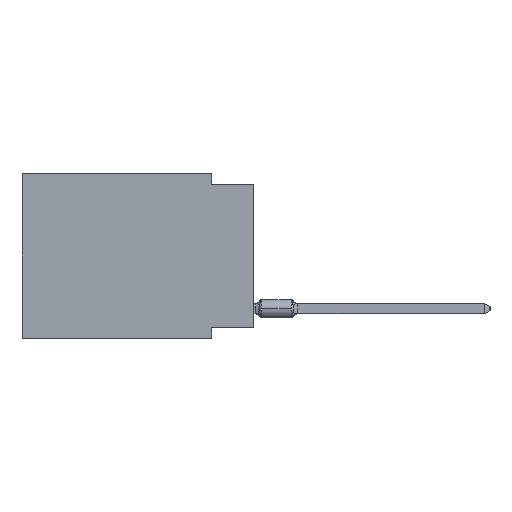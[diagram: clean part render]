
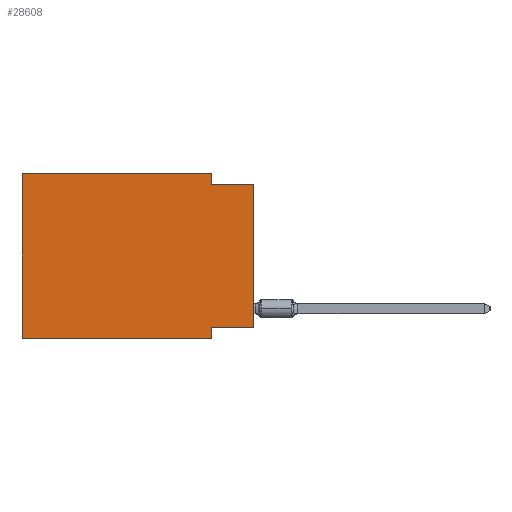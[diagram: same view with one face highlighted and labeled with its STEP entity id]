
A CAD part, left-side view. The second image highlights one B-rep face of the part: STEP entity #28608.
In plain terms, the highlighted planar face has unit normal (-1, 0, 0).
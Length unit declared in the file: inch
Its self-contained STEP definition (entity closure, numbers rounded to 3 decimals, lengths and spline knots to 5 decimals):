
#1460 = ORIENTED_EDGE ( 'NONE', *, *, #8875, .F. ) ;
#2467 = CARTESIAN_POINT ( 'NONE',  ( 0., 0.1, 0. ) ) ;
#2951 = VECTOR ( 'NONE', #33342, 39.37008 ) ;
#3964 = ORIENTED_EDGE ( 'NONE', *, *, #6357, .T. ) ;
#4202 = DIRECTION ( 'NONE',  ( 0., -1., 0. ) ) ;
#4640 = VECTOR ( 'NONE', #26153, 39.37008 ) ;
#4978 = VERTEX_POINT ( 'NONE', #22599 ) ;
#5071 = CARTESIAN_POINT ( 'NONE',  ( 0., 0.1, -0.39 ) ) ;
#5503 = LINE ( 'NONE', #30971, #20726 ) ;
#5688 = VECTOR ( 'NONE', #14243, 39.37008 ) ;
#6357 = EDGE_CURVE ( 'NONE', #12077, #12514, #19902, .T. ) ;
#6684 = CARTESIAN_POINT ( 'NONE',  ( 0., 0.55, 0. ) ) ;
#7269 = LINE ( 'NONE', #5071, #28558 ) ;
#7432 = PLANE ( 'NONE',  #23511 ) ;
#7542 = CARTESIAN_POINT ( 'NONE',  ( 0., 0.1, -0.39 ) ) ;
#7675 = ORIENTED_EDGE ( 'NONE', *, *, #27380, .F. ) ;
#8429 = CARTESIAN_POINT ( 'NONE',  ( 0., 0., -0.365 ) ) ;
#8778 = LINE ( 'NONE', #22241, #9567 ) ;
#8875 = EDGE_CURVE ( 'NONE', #13925, #28356, #27230, .T. ) ;
#9567 = VECTOR ( 'NONE', #32204, 39.37008 ) ;
#9795 = CARTESIAN_POINT ( 'NONE',  ( 0., 0.55, 0. ) ) ;
#10225 = ORIENTED_EDGE ( 'NONE', *, *, #12659, .T. ) ;
#10295 = DIRECTION ( 'NONE',  ( 0., 0., -1. ) ) ;
#10405 = ORIENTED_EDGE ( 'NONE', *, *, #28668, .F. ) ;
#10538 = CARTESIAN_POINT ( 'NONE',  ( 0., 0., -0.025 ) ) ;
#10794 = EDGE_CURVE ( 'NONE', #19564, #29018, #8778, .T. ) ;
#11011 = CARTESIAN_POINT ( 'NONE',  ( 0., 0.55, -0.39 ) ) ;
#12077 = VERTEX_POINT ( 'NONE', #11011 ) ;
#12514 = VERTEX_POINT ( 'NONE', #7542 ) ;
#12576 = VECTOR ( 'NONE', #4202, 39.37008 ) ;
#12659 = EDGE_CURVE ( 'NONE', #4978, #28356, #5503, .T. ) ;
#13331 = LINE ( 'NONE', #8429, #4640 ) ;
#13606 = CARTESIAN_POINT ( 'NONE',  ( 0., 0.55, 0. ) ) ;
#13925 = VERTEX_POINT ( 'NONE', #26215 ) ;
#13953 = LINE ( 'NONE', #13606, #26763 ) ;
#14243 = DIRECTION ( 'NONE',  ( 0., -1., 0. ) ) ;
#14896 = VERTEX_POINT ( 'NONE', #31505 ) ;
#15834 = ORIENTED_EDGE ( 'NONE', *, *, #10794, .F. ) ;
#15968 = DIRECTION ( 'NONE',  ( 0., 0., 1. ) ) ;
#16368 = EDGE_CURVE ( 'NONE', #12077, #19564, #13953, .T. ) ;
#17104 = CARTESIAN_POINT ( 'NONE',  ( 0., 0., -0.025 ) ) ;
#17888 = FACE_OUTER_BOUND ( 'NONE', #33219, .T. ) ;
#19564 = VERTEX_POINT ( 'NONE', #6684 ) ;
#19902 = LINE ( 'NONE', #27339, #12576 ) ;
#20713 = LINE ( 'NONE', #33001, #2951 ) ;
#20726 = VECTOR ( 'NONE', #31316, 39.37008 ) ;
#22241 = CARTESIAN_POINT ( 'NONE',  ( 0., 0.55, 0. ) ) ;
#22428 = DIRECTION ( 'NONE',  ( 1., 0., 0. ) ) ;
#22599 = CARTESIAN_POINT ( 'NONE',  ( 0., 0., -0.365 ) ) ;
#22617 = DIRECTION ( 'NONE',  ( 0., 0., -1. ) ) ;
#23511 = AXIS2_PLACEMENT_3D ( 'NONE', #9795, #22428, #10295 ) ;
#24018 = ORIENTED_EDGE ( 'NONE', *, *, #32640, .F. ) ;
#26153 = DIRECTION ( 'NONE',  ( 0., 1., 0. ) ) ;
#26215 = CARTESIAN_POINT ( 'NONE',  ( 0., 0.1, -0.025 ) ) ;
#26763 = VECTOR ( 'NONE', #15968, 39.37008 ) ;
#27230 = LINE ( 'NONE', #17104, #5688 ) ;
#27339 = CARTESIAN_POINT ( 'NONE',  ( 0., 0.55, -0.39 ) ) ;
#27380 = EDGE_CURVE ( 'NONE', #29018, #13925, #20713, .T. ) ;
#27646 = ORIENTED_EDGE ( 'NONE', *, *, #16368, .F. ) ;
#28356 = VERTEX_POINT ( 'NONE', #10538 ) ;
#28558 = VECTOR ( 'NONE', #22617, 39.37008 ) ;
#28608 = ADVANCED_FACE ( 'NONE', ( #17888 ), #7432, .F. ) ;
#28668 = EDGE_CURVE ( 'NONE', #4978, #14896, #13331, .T. ) ;
#29018 = VERTEX_POINT ( 'NONE', #2467 ) ;
#30971 = CARTESIAN_POINT ( 'NONE',  ( 0., 0., 0. ) ) ;
#31316 = DIRECTION ( 'NONE',  ( 0., 0., 1. ) ) ;
#31505 = CARTESIAN_POINT ( 'NONE',  ( 0., 0.1, -0.365 ) ) ;
#32204 = DIRECTION ( 'NONE',  ( 0., -1., 0. ) ) ;
#32640 = EDGE_CURVE ( 'NONE', #14896, #12514, #7269, .T. ) ;
#33001 = CARTESIAN_POINT ( 'NONE',  ( 0., 0.1, 0. ) ) ;
#33219 = EDGE_LOOP ( 'NONE', ( #10225, #1460, #7675, #15834, #27646, #3964, #24018, #10405 ) ) ;
#33342 = DIRECTION ( 'NONE',  ( 0., 0., -1. ) ) ;
